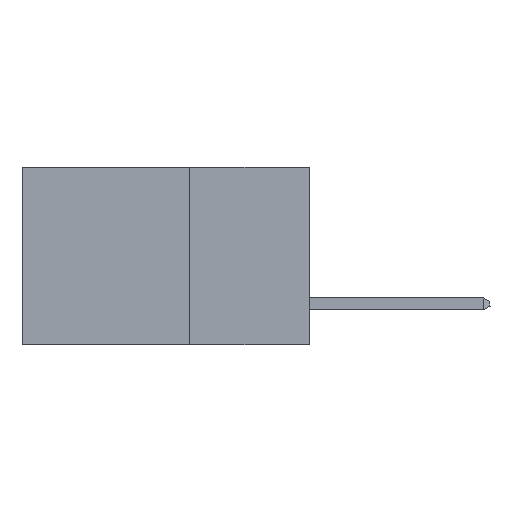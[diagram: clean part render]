
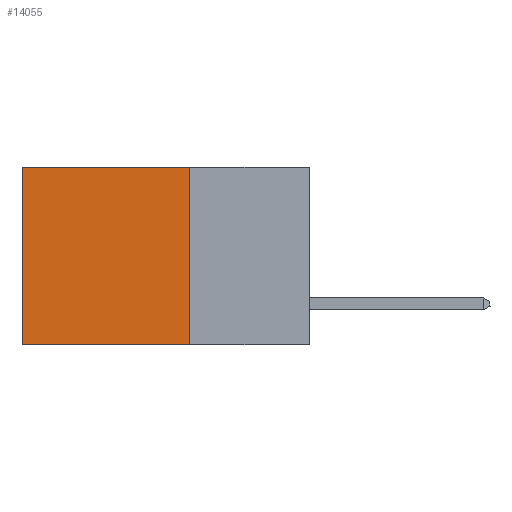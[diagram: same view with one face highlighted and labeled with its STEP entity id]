
A CAD part, left-side view. The second image highlights one B-rep face of the part: STEP entity #14055.
In plain terms, the highlighted planar face has unit normal (-1, 0, 0).
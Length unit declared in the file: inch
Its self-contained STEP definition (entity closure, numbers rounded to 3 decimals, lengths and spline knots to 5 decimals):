
#1289 = DIRECTION ( 'NONE',  ( 0., 1., 0. ) ) ;
#1688 = CARTESIAN_POINT ( 'NONE',  ( 0.2875, 0.25, 0. ) ) ;
#2393 = CARTESIAN_POINT ( 'NONE',  ( 0.2875, 0.6, 0. ) ) ;
#6465 = VERTEX_POINT ( 'NONE', #45382 ) ;
#6936 = VECTOR ( 'NONE', #30159, 39.37008 ) ;
#7163 = FACE_OUTER_BOUND ( 'NONE', #31500, .T. ) ;
#8745 = AXIS2_PLACEMENT_3D ( 'NONE', #31925, #14979, #38028 ) ;
#9109 = LINE ( 'NONE', #22985, #37470 ) ;
#9374 = PLANE ( 'NONE',  #8745 ) ;
#11114 = EDGE_CURVE ( 'NONE', #6465, #21067, #9109, .T. ) ;
#11794 = VECTOR ( 'NONE', #25689, 39.37008 ) ;
#12006 = EDGE_CURVE ( 'NONE', #42824, #20688, #40853, .T. ) ;
#12216 = DIRECTION ( 'NONE',  ( 0., 0., -1. ) ) ;
#13545 = EDGE_CURVE ( 'NONE', #6465, #42824, #36725, .T. ) ;
#14055 = ADVANCED_FACE ( 'NONE', ( #7163 ), #9374, .F. ) ;
#14979 = DIRECTION ( 'NONE',  ( 1., 0., 0. ) ) ;
#15688 = ORIENTED_EDGE ( 'NONE', *, *, #13545, .F. ) ;
#19312 = CARTESIAN_POINT ( 'NONE',  ( 0.2875, 0.6, -0.37 ) ) ;
#20688 = VERTEX_POINT ( 'NONE', #19312 ) ;
#21067 = VERTEX_POINT ( 'NONE', #2393 ) ;
#22985 = CARTESIAN_POINT ( 'NONE',  ( 0.2875, 0.25, 0. ) ) ;
#25689 = DIRECTION ( 'NONE',  ( 0., 1., 0. ) ) ;
#30159 = DIRECTION ( 'NONE',  ( 0., 0., -1. ) ) ;
#30864 = ORIENTED_EDGE ( 'NONE', *, *, #32648, .T. ) ;
#31500 = EDGE_LOOP ( 'NONE', ( #30864, #42177, #15688, #45617 ) ) ;
#31649 = CARTESIAN_POINT ( 'NONE',  ( 0.2875, 0.25, -0.37 ) ) ;
#31925 = CARTESIAN_POINT ( 'NONE',  ( 0.2875, 0.25, 0. ) ) ;
#32648 = EDGE_CURVE ( 'NONE', #21067, #20688, #46137, .T. ) ;
#33199 = CARTESIAN_POINT ( 'NONE',  ( 0.2875, 0.6, 0. ) ) ;
#36725 = LINE ( 'NONE', #1688, #43580 ) ;
#37470 = VECTOR ( 'NONE', #1289, 39.37008 ) ;
#38028 = DIRECTION ( 'NONE',  ( 0., 0., -1. ) ) ;
#40853 = LINE ( 'NONE', #31649, #11794 ) ;
#42177 = ORIENTED_EDGE ( 'NONE', *, *, #12006, .F. ) ;
#42824 = VERTEX_POINT ( 'NONE', #46480 ) ;
#43580 = VECTOR ( 'NONE', #12216, 39.37008 ) ;
#45382 = CARTESIAN_POINT ( 'NONE',  ( 0.2875, 0.25, 0. ) ) ;
#45617 = ORIENTED_EDGE ( 'NONE', *, *, #11114, .T. ) ;
#46137 = LINE ( 'NONE', #33199, #6936 ) ;
#46480 = CARTESIAN_POINT ( 'NONE',  ( 0.2875, 0.25, -0.37 ) ) ;
